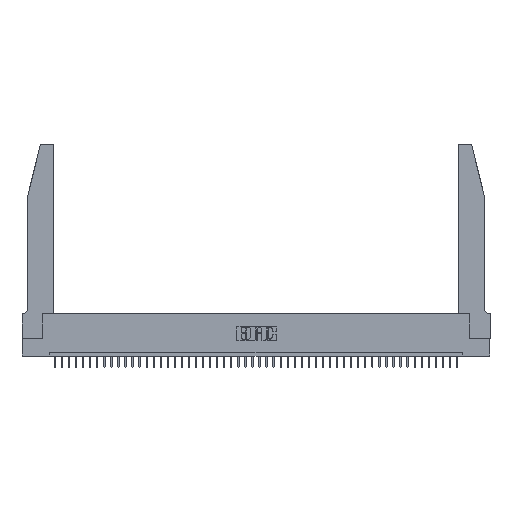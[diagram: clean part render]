
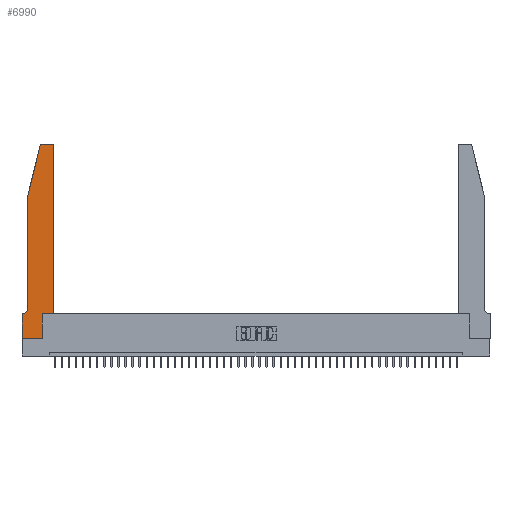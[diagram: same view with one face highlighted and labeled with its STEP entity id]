
A CAD part, top view. The second image highlights one B-rep face of the part: STEP entity #6990.
In plain terms, the highlighted planar face has unit normal (0, 0, 1).
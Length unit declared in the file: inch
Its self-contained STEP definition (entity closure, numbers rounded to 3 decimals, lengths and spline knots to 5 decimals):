
#489 = VERTEX_POINT ( 'NONE', #17410 ) ;
#1202 = CARTESIAN_POINT ( 'NONE',  ( 0.25487, 2.72718, 0.37 ) ) ;
#1748 = EDGE_CURVE ( 'NONE', #22789, #14322, #35742, .T. ) ;
#1926 = CARTESIAN_POINT ( 'NONE',  ( 0.4505, 0.35, 0.37 ) ) ;
#2588 = AXIS2_PLACEMENT_3D ( 'NONE', #17258, #20868, #28066 ) ;
#3065 = VECTOR ( 'NONE', #45110, 39.37008 ) ;
#3863 = AXIS2_PLACEMENT_3D ( 'NONE', #32647, #30761, #20123 ) ;
#3864 = CIRCLE ( 'NONE', #2588, 0.07 ) ;
#4631 = CARTESIAN_POINT ( 'NONE',  ( 0.0755, 0.42, 0.37 ) ) ;
#6383 = ORIENTED_EDGE ( 'NONE', *, *, #1748, .T. ) ;
#6677 = LINE ( 'NONE', #36756, #34070 ) ;
#6990 = ADVANCED_FACE ( 'NONE', ( #27649 ), #36089, .T. ) ;
#8129 = VECTOR ( 'NONE', #37161, 39.37008 ) ;
#8216 = VECTOR ( 'NONE', #44087, 39.37008 ) ;
#9603 = ORIENTED_EDGE ( 'NONE', *, *, #42049, .T. ) ;
#11706 = CARTESIAN_POINT ( 'NONE',  ( 0.4505, 0.35, 0.37 ) ) ;
#12184 = CARTESIAN_POINT ( 'NONE',  ( 0.4505, 0.35, 0.37 ) ) ;
#12324 = VERTEX_POINT ( 'NONE', #29955 ) ;
#13105 = CARTESIAN_POINT ( 'NONE',  ( 0.0055, 0.35, 0.37 ) ) ;
#13663 = DIRECTION ( 'NONE',  ( 0., 0., 1. ) ) ;
#14295 = ORIENTED_EDGE ( 'NONE', *, *, #22918, .T. ) ;
#14322 = VERTEX_POINT ( 'NONE', #1202 ) ;
#14609 = LINE ( 'NONE', #19943, #37007 ) ;
#14891 = VECTOR ( 'NONE', #20784, 39.37008 ) ;
#15285 = DIRECTION ( 'NONE',  ( -1., 0., 0. ) ) ;
#15500 = CARTESIAN_POINT ( 'NONE',  ( 0.0755, 2., 0.37 ) ) ;
#15901 = LINE ( 'NONE', #27046, #19830 ) ;
#16113 = DIRECTION ( 'NONE',  ( -1., 0., 0. ) ) ;
#17258 = CARTESIAN_POINT ( 'NONE',  ( 0.0055, 0.42, 0.37 ) ) ;
#17410 = CARTESIAN_POINT ( 'NONE',  ( 0.4505, 2.72, 0.37 ) ) ;
#17960 = EDGE_CURVE ( 'NONE', #489, #24205, #35894, .T. ) ;
#18083 = VECTOR ( 'NONE', #19936, 39.37008 ) ;
#18133 = CARTESIAN_POINT ( 'NONE',  ( 0.284, 2.72, 0.37 ) ) ;
#18513 = ORIENTED_EDGE ( 'NONE', *, *, #29333, .T. ) ;
#19780 = VERTEX_POINT ( 'NONE', #11706 ) ;
#19830 = VECTOR ( 'NONE', #16113, 39.37008 ) ;
#19936 = DIRECTION ( 'NONE',  ( 1., 0., 0. ) ) ;
#19943 = CARTESIAN_POINT ( 'NONE',  ( 0., 0., 0.37 ) ) ;
#20103 = CARTESIAN_POINT ( 'NONE',  ( 0., 0.35, 0.37 ) ) ;
#20115 = ORIENTED_EDGE ( 'NONE', *, *, #39268, .T. ) ;
#20123 = DIRECTION ( 'NONE',  ( 1., 0., 0. ) ) ;
#20784 = DIRECTION ( 'NONE',  ( 0., -1., 0. ) ) ;
#20839 = ORIENTED_EDGE ( 'NONE', *, *, #35225, .T. ) ;
#20868 = DIRECTION ( 'NONE',  ( 0., 0., -1. ) ) ;
#21410 = ORIENTED_EDGE ( 'NONE', *, *, #24199, .T. ) ;
#21427 = VERTEX_POINT ( 'NONE', #35667 ) ;
#21829 = EDGE_CURVE ( 'NONE', #19780, #489, #32754, .T. ) ;
#22647 = VERTEX_POINT ( 'NONE', #43254 ) ;
#22789 = VERTEX_POINT ( 'NONE', #46034 ) ;
#22918 = EDGE_CURVE ( 'NONE', #14322, #29033, #37315, .T. ) ;
#23726 = LINE ( 'NONE', #30607, #3065 ) ;
#24199 = EDGE_CURVE ( 'NONE', #21427, #22647, #45239, .T. ) ;
#24205 = VERTEX_POINT ( 'NONE', #26833 ) ;
#24672 = ORIENTED_EDGE ( 'NONE', *, *, #36985, .T. ) ;
#26059 = CARTESIAN_POINT ( 'NONE',  ( 0.2865, 0.35, 0.37 ) ) ;
#26428 = ORIENTED_EDGE ( 'NONE', *, *, #17960, .T. ) ;
#26759 = VECTOR ( 'NONE', #39827, 39.37008 ) ;
#26833 = CARTESIAN_POINT ( 'NONE',  ( 0.4205, 2.75, 0.37 ) ) ;
#26964 = CARTESIAN_POINT ( 'NONE',  ( 0.0755, 2., 0.37 ) ) ;
#27046 = CARTESIAN_POINT ( 'NONE',  ( 0.0755, 0.35, 0.37 ) ) ;
#27649 = FACE_OUTER_BOUND ( 'NONE', #30936, .T. ) ;
#27862 = EDGE_CURVE ( 'NONE', #22647, #19780, #45522, .T. ) ;
#28066 = DIRECTION ( 'NONE',  ( -1., 0., 0. ) ) ;
#29033 = VERTEX_POINT ( 'NONE', #26964 ) ;
#29333 = EDGE_CURVE ( 'NONE', #12324, #21427, #23726, .T. ) ;
#29955 = CARTESIAN_POINT ( 'NONE',  ( 0., 0., 0.37 ) ) ;
#30607 = CARTESIAN_POINT ( 'NONE',  ( 0., 0., 0.37 ) ) ;
#30761 = DIRECTION ( 'NONE',  ( 0., 0., 1. ) ) ;
#30936 = EDGE_LOOP ( 'NONE', ( #20839, #6383, #14295, #9603, #35386, #24672, #20115, #18513, #21410, #41603, #31966, #26428 ) ) ;
#31966 = ORIENTED_EDGE ( 'NONE', *, *, #21829, .T. ) ;
#32647 = CARTESIAN_POINT ( 'NONE',  ( 0., 0.35, 0.37 ) ) ;
#32754 = LINE ( 'NONE', #12184, #8129 ) ;
#32853 = DIRECTION ( 'NONE',  ( 1., 0., 0. ) ) ;
#34070 = VECTOR ( 'NONE', #15285, 39.37008 ) ;
#34919 = EDGE_CURVE ( 'NONE', #35765, #40891, #3864, .T. ) ;
#35071 = CARTESIAN_POINT ( 'NONE',  ( 0.4205, 2.72, 0.37 ) ) ;
#35225 = EDGE_CURVE ( 'NONE', #24205, #22789, #6677, .T. ) ;
#35386 = ORIENTED_EDGE ( 'NONE', *, *, #34919, .T. ) ;
#35667 = CARTESIAN_POINT ( 'NONE',  ( 0.2865, 0., 0.37 ) ) ;
#35742 = CIRCLE ( 'NONE', #35795, 0.03 ) ;
#35765 = VERTEX_POINT ( 'NONE', #4631 ) ;
#35795 = AXIS2_PLACEMENT_3D ( 'NONE', #18133, #36144, #32853 ) ;
#35894 = CIRCLE ( 'NONE', #40248, 0.03 ) ;
#36089 = PLANE ( 'NONE',  #3863 ) ;
#36144 = DIRECTION ( 'NONE',  ( 0., 0., 1. ) ) ;
#36401 = DIRECTION ( 'NONE',  ( 1., 0., 0. ) ) ;
#36736 = LINE ( 'NONE', #45624, #14891 ) ;
#36756 = CARTESIAN_POINT ( 'NONE',  ( 0.2605, 2.75, 0.37 ) ) ;
#36985 = EDGE_CURVE ( 'NONE', #40891, #39263, #15901, .T. ) ;
#37007 = VECTOR ( 'NONE', #41203, 39.37008 ) ;
#37161 = DIRECTION ( 'NONE',  ( 0., 1., 0. ) ) ;
#37315 = LINE ( 'NONE', #15500, #8216 ) ;
#39263 = VERTEX_POINT ( 'NONE', #20103 ) ;
#39268 = EDGE_CURVE ( 'NONE', #39263, #12324, #14609, .T. ) ;
#39827 = DIRECTION ( 'NONE',  ( 0., 1., 0. ) ) ;
#40248 = AXIS2_PLACEMENT_3D ( 'NONE', #35071, #13663, #36401 ) ;
#40891 = VERTEX_POINT ( 'NONE', #13105 ) ;
#41203 = DIRECTION ( 'NONE',  ( 0., -1., 0. ) ) ;
#41603 = ORIENTED_EDGE ( 'NONE', *, *, #27862, .T. ) ;
#42049 = EDGE_CURVE ( 'NONE', #29033, #35765, #36736, .T. ) ;
#43254 = CARTESIAN_POINT ( 'NONE',  ( 0.2865, 0.35, 0.37 ) ) ;
#44087 = DIRECTION ( 'NONE',  ( -0.239, -0.971, 0. ) ) ;
#45110 = DIRECTION ( 'NONE',  ( 1., 0., 0. ) ) ;
#45239 = LINE ( 'NONE', #26059, #26759 ) ;
#45522 = LINE ( 'NONE', #1926, #18083 ) ;
#45624 = CARTESIAN_POINT ( 'NONE',  ( 0.0755, 2., 0.37 ) ) ;
#46034 = CARTESIAN_POINT ( 'NONE',  ( 0.284, 2.75, 0.37 ) ) ;
